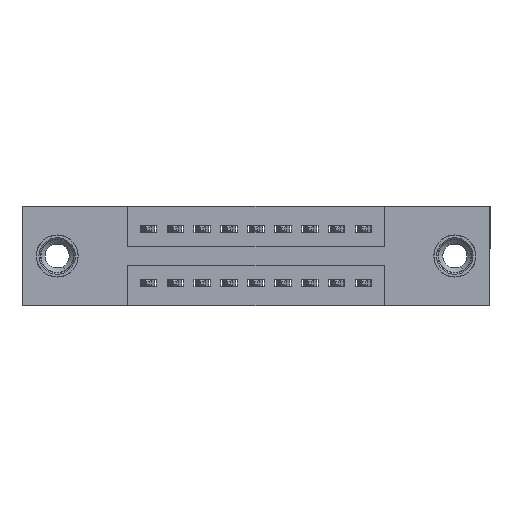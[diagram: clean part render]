
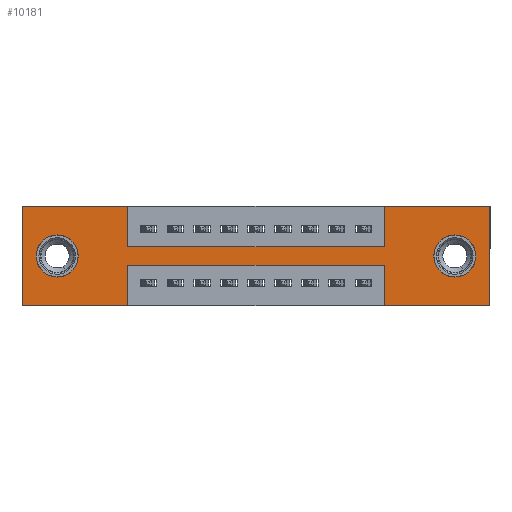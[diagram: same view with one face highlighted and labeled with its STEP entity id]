
A CAD part, front view. The second image highlights one B-rep face of the part: STEP entity #10181.
In plain terms, the highlighted planar face has unit normal (0, -1, 0).
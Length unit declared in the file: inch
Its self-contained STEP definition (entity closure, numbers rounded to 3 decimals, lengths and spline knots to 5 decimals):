
#186 = CIRCLE ( 'NONE', #15289, 0.078 ) ;
#239 = CARTESIAN_POINT ( 'NONE',  ( 0.13, 0., -0.185 ) ) ;
#244 = CARTESIAN_POINT ( 'NONE',  ( 1.605, 0., -0.263 ) ) ;
#390 = VECTOR ( 'NONE', #3540, 39.37008 ) ;
#586 = FACE_BOUND ( 'NONE', #14904, .T. ) ;
#758 = DIRECTION ( 'NONE',  ( 0., 0., 1. ) ) ;
#1096 = ORIENTED_EDGE ( 'NONE', *, *, #1113, .F. ) ;
#1113 = EDGE_CURVE ( 'NONE', #14923, #4125, #14538, .T. ) ;
#1199 = CARTESIAN_POINT ( 'NONE',  ( 1.3425, 0., -0.37 ) ) ;
#1308 = EDGE_CURVE ( 'NONE', #6532, #11683, #7705, .T. ) ;
#1342 = ORIENTED_EDGE ( 'NONE', *, *, #11011, .F. ) ;
#1532 = EDGE_CURVE ( 'NONE', #14345, #4065, #12168, .T. ) ;
#1749 = PLANE ( 'NONE',  #13840 ) ;
#1964 = CARTESIAN_POINT ( 'NONE',  ( 0.3925, 0., 0. ) ) ;
#2128 = VERTEX_POINT ( 'NONE', #1964 ) ;
#2265 = DIRECTION ( 'NONE',  ( -1., 0., 0. ) ) ;
#2539 = DIRECTION ( 'NONE',  ( 0., 0., 1. ) ) ;
#2724 = ORIENTED_EDGE ( 'NONE', *, *, #15463, .F. ) ;
#2805 = AXIS2_PLACEMENT_3D ( 'NONE', #16092, #16153, #5101 ) ;
#3007 = CARTESIAN_POINT ( 'NONE',  ( 0.3925, 0., -0.37 ) ) ;
#3321 = FACE_OUTER_BOUND ( 'NONE', #10890, .T. ) ;
#3529 = AXIS2_PLACEMENT_3D ( 'NONE', #15522, #14352, #10665 ) ;
#3540 = DIRECTION ( 'NONE',  ( 0., 0., -1. ) ) ;
#3575 = VERTEX_POINT ( 'NONE', #244 ) ;
#3803 = CARTESIAN_POINT ( 'NONE',  ( 1.3425, 0., -0.15 ) ) ;
#4065 = VERTEX_POINT ( 'NONE', #13194 ) ;
#4125 = VERTEX_POINT ( 'NONE', #7561 ) ;
#4323 = VECTOR ( 'NONE', #2265, 39.37008 ) ;
#4341 = FACE_BOUND ( 'NONE', #7717, .T. ) ;
#4639 = LINE ( 'NONE', #9791, #6835 ) ;
#4645 = DIRECTION ( 'NONE',  ( 1., 0., 0. ) ) ;
#4919 = ORIENTED_EDGE ( 'NONE', *, *, #10932, .T. ) ;
#5022 = CARTESIAN_POINT ( 'NONE',  ( 1.605, 0., -0.185 ) ) ;
#5100 = CARTESIAN_POINT ( 'NONE',  ( 1.735, 0., 0. ) ) ;
#5101 = DIRECTION ( 'NONE',  ( 0., 0., -1. ) ) ;
#5143 = CIRCLE ( 'NONE', #3529, 0.078 ) ;
#5184 = ORIENTED_EDGE ( 'NONE', *, *, #14931, .T. ) ;
#5253 = CARTESIAN_POINT ( 'NONE',  ( 1.3425, 0., -0.37 ) ) ;
#5395 = CARTESIAN_POINT ( 'NONE',  ( 0.3925, 0., -0.15 ) ) ;
#5450 = VERTEX_POINT ( 'NONE', #15217 ) ;
#5465 = ORIENTED_EDGE ( 'NONE', *, *, #1532, .F. ) ;
#5759 = EDGE_CURVE ( 'NONE', #3575, #11168, #6452, .T. ) ;
#5790 = EDGE_CURVE ( 'NONE', #10327, #10721, #4639, .T. ) ;
#5853 = ORIENTED_EDGE ( 'NONE', *, *, #10300, .F. ) ;
#5872 = EDGE_CURVE ( 'NONE', #11168, #3575, #12304, .T. ) ;
#5965 = ORIENTED_EDGE ( 'NONE', *, *, #6515, .F. ) ;
#5988 = AXIS2_PLACEMENT_3D ( 'NONE', #5022, #13829, #15142 ) ;
#6367 = VECTOR ( 'NONE', #9988, 39.37008 ) ;
#6452 = CIRCLE ( 'NONE', #2805, 0.078 ) ;
#6515 = EDGE_CURVE ( 'NONE', #11683, #10670, #16241, .T. ) ;
#6532 = VERTEX_POINT ( 'NONE', #15041 ) ;
#6600 = CARTESIAN_POINT ( 'NONE',  ( 0.3925, 0., -0.37 ) ) ;
#6835 = VECTOR ( 'NONE', #14807, 39.37008 ) ;
#6848 = DIRECTION ( 'NONE',  ( 0., -1., 0. ) ) ;
#6854 = ORIENTED_EDGE ( 'NONE', *, *, #13630, .F. ) ;
#7005 = CARTESIAN_POINT ( 'NONE',  ( 0., 0., 0. ) ) ;
#7094 = CARTESIAN_POINT ( 'NONE',  ( 1.735, 0., -0.37 ) ) ;
#7199 = CARTESIAN_POINT ( 'NONE',  ( 0., 0., -0.37 ) ) ;
#7393 = ORIENTED_EDGE ( 'NONE', *, *, #9347, .F. ) ;
#7545 = CARTESIAN_POINT ( 'NONE',  ( 0.3925, 0., 0. ) ) ;
#7561 = CARTESIAN_POINT ( 'NONE',  ( 0.3925, 0., -0.22 ) ) ;
#7705 = LINE ( 'NONE', #5100, #13980 ) ;
#7717 = EDGE_LOOP ( 'NONE', ( #11063, #16038 ) ) ;
#7809 = DIRECTION ( 'NONE',  ( 0., 0., -1. ) ) ;
#8288 = CARTESIAN_POINT ( 'NONE',  ( 1.3425, 0., 0. ) ) ;
#8333 = VECTOR ( 'NONE', #4645, 39.37008 ) ;
#8838 = DIRECTION ( 'NONE',  ( -1., 0., 0. ) ) ;
#8917 = DIRECTION ( 'NONE',  ( 1., 0., 0. ) ) ;
#8962 = LINE ( 'NONE', #5395, #8333 ) ;
#8997 = ORIENTED_EDGE ( 'NONE', *, *, #1308, .F. ) ;
#9233 = ORIENTED_EDGE ( 'NONE', *, *, #5790, .F. ) ;
#9248 = DIRECTION ( 'NONE',  ( 0., 0., -1. ) ) ;
#9272 = VECTOR ( 'NONE', #9248, 39.37008 ) ;
#9319 = CARTESIAN_POINT ( 'NONE',  ( 1.3425, 0., -0.22 ) ) ;
#9347 = EDGE_CURVE ( 'NONE', #10721, #2128, #12410, .T. ) ;
#9665 = LINE ( 'NONE', #7545, #390 ) ;
#9700 = VERTEX_POINT ( 'NONE', #12500 ) ;
#9791 = CARTESIAN_POINT ( 'NONE',  ( 0., 0., 0. ) ) ;
#9849 = CARTESIAN_POINT ( 'NONE',  ( 0.3925, 0., -0.22 ) ) ;
#9988 = DIRECTION ( 'NONE',  ( 0., 0., 1. ) ) ;
#10057 = VECTOR ( 'NONE', #758, 39.37008 ) ;
#10094 = LINE ( 'NONE', #1199, #6367 ) ;
#10181 = ADVANCED_FACE ( 'NONE', ( #4341, #586, #3321 ), #1749, .T. ) ;
#10300 = EDGE_CURVE ( 'NONE', #2128, #11069, #9665, .T. ) ;
#10307 = DIRECTION ( 'NONE',  ( 0., 1., 0. ) ) ;
#10327 = VERTEX_POINT ( 'NONE', #11510 ) ;
#10599 = LINE ( 'NONE', #6600, #9272 ) ;
#10665 = DIRECTION ( 'NONE',  ( 0., 0., 1. ) ) ;
#10670 = VERTEX_POINT ( 'NONE', #5253 ) ;
#10721 = VERTEX_POINT ( 'NONE', #7005 ) ;
#10869 = DIRECTION ( 'NONE',  ( 1., 0., 0. ) ) ;
#10890 = EDGE_LOOP ( 'NONE', ( #1342, #1096, #13042, #5965, #8997, #14369, #5465, #6854, #5853, #7393, #9233, #2724 ) ) ;
#10932 = EDGE_CURVE ( 'NONE', #9700, #5450, #186, .T. ) ;
#11011 = EDGE_CURVE ( 'NONE', #4125, #14566, #10599, .T. ) ;
#11063 = ORIENTED_EDGE ( 'NONE', *, *, #5872, .T. ) ;
#11069 = VERTEX_POINT ( 'NONE', #12795 ) ;
#11168 = VERTEX_POINT ( 'NONE', #11998 ) ;
#11207 = VECTOR ( 'NONE', #10869, 39.37008 ) ;
#11510 = CARTESIAN_POINT ( 'NONE',  ( 0., 0., -0.37 ) ) ;
#11683 = VERTEX_POINT ( 'NONE', #7094 ) ;
#11993 = CARTESIAN_POINT ( 'NONE',  ( 0., 0., 0. ) ) ;
#11998 = CARTESIAN_POINT ( 'NONE',  ( 1.605, 0., -0.107 ) ) ;
#12009 = VECTOR ( 'NONE', #8917, 39.37008 ) ;
#12168 = LINE ( 'NONE', #8288, #10057 ) ;
#12304 = CIRCLE ( 'NONE', #5988, 0.078 ) ;
#12410 = LINE ( 'NONE', #16242, #12009 ) ;
#12500 = CARTESIAN_POINT ( 'NONE',  ( 0.13, 0., -0.107 ) ) ;
#12792 = LINE ( 'NONE', #15171, #13013 ) ;
#12795 = CARTESIAN_POINT ( 'NONE',  ( 0.3925, 0., -0.15 ) ) ;
#13013 = VECTOR ( 'NONE', #8838, 39.37008 ) ;
#13042 = ORIENTED_EDGE ( 'NONE', *, *, #14390, .F. ) ;
#13194 = CARTESIAN_POINT ( 'NONE',  ( 1.3425, 0., 0. ) ) ;
#13200 = DIRECTION ( 'NONE',  ( 0., 0., -1. ) ) ;
#13277 = VECTOR ( 'NONE', #13560, 39.37008 ) ;
#13560 = DIRECTION ( 'NONE',  ( -1., 0., 0. ) ) ;
#13630 = EDGE_CURVE ( 'NONE', #11069, #14345, #8962, .T. ) ;
#13829 = DIRECTION ( 'NONE',  ( 0., 1., 0. ) ) ;
#13840 = AXIS2_PLACEMENT_3D ( 'NONE', #15722, #6848, #13200 ) ;
#13980 = VECTOR ( 'NONE', #7809, 39.37008 ) ;
#14345 = VERTEX_POINT ( 'NONE', #3803 ) ;
#14352 = DIRECTION ( 'NONE',  ( 0., 1., 0. ) ) ;
#14369 = ORIENTED_EDGE ( 'NONE', *, *, #15101, .F. ) ;
#14390 = EDGE_CURVE ( 'NONE', #10670, #14923, #10094, .T. ) ;
#14538 = LINE ( 'NONE', #9849, #4323 ) ;
#14550 = LINE ( 'NONE', #11993, #11207 ) ;
#14566 = VERTEX_POINT ( 'NONE', #3007 ) ;
#14807 = DIRECTION ( 'NONE',  ( 0., 0., 1. ) ) ;
#14904 = EDGE_LOOP ( 'NONE', ( #4919, #5184 ) ) ;
#14923 = VERTEX_POINT ( 'NONE', #9319 ) ;
#14931 = EDGE_CURVE ( 'NONE', #5450, #9700, #5143, .T. ) ;
#15041 = CARTESIAN_POINT ( 'NONE',  ( 1.735, 0., 0. ) ) ;
#15101 = EDGE_CURVE ( 'NONE', #4065, #6532, #14550, .T. ) ;
#15142 = DIRECTION ( 'NONE',  ( 0., 0., -1. ) ) ;
#15171 = CARTESIAN_POINT ( 'NONE',  ( 0., 0., -0.37 ) ) ;
#15217 = CARTESIAN_POINT ( 'NONE',  ( 0.13, 0., -0.263 ) ) ;
#15289 = AXIS2_PLACEMENT_3D ( 'NONE', #239, #10307, #2539 ) ;
#15463 = EDGE_CURVE ( 'NONE', #14566, #10327, #12792, .T. ) ;
#15522 = CARTESIAN_POINT ( 'NONE',  ( 0.13, 0., -0.185 ) ) ;
#15722 = CARTESIAN_POINT ( 'NONE',  ( 0., 0., -0.37 ) ) ;
#16038 = ORIENTED_EDGE ( 'NONE', *, *, #5759, .T. ) ;
#16092 = CARTESIAN_POINT ( 'NONE',  ( 1.605, 0., -0.185 ) ) ;
#16153 = DIRECTION ( 'NONE',  ( 0., 1., 0. ) ) ;
#16241 = LINE ( 'NONE', #7199, #13277 ) ;
#16242 = CARTESIAN_POINT ( 'NONE',  ( 0., 0., 0. ) ) ;
